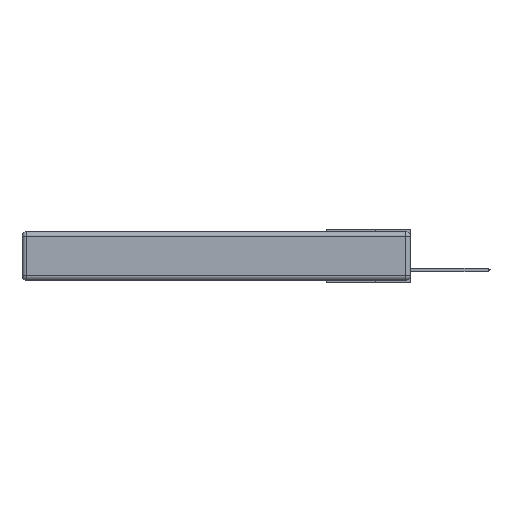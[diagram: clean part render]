
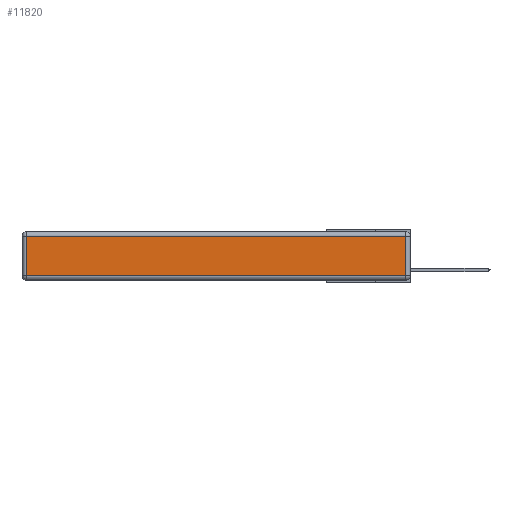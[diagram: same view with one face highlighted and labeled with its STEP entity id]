
A CAD part, left-side view. The second image highlights one B-rep face of the part: STEP entity #11820.
In plain terms, the highlighted planar face has unit normal (-1, 0, 0).
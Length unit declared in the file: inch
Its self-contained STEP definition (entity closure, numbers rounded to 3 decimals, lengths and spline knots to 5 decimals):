
#260 = VECTOR ( 'NONE', #11265, 39.37008 ) ;
#859 = CARTESIAN_POINT ( 'NONE',  ( 0., 0., -0.343 ) ) ;
#1187 = ORIENTED_EDGE ( 'NONE', *, *, #10939, .T. ) ;
#1358 = VECTOR ( 'NONE', #7490, 39.37008 ) ;
#1414 = CARTESIAN_POINT ( 'NONE',  ( 0., 2.72, -0.313 ) ) ;
#1462 = VERTEX_POINT ( 'NONE', #13687 ) ;
#1699 = LINE ( 'NONE', #4049, #10821 ) ;
#2009 = VERTEX_POINT ( 'NONE', #2602 ) ;
#2602 = CARTESIAN_POINT ( 'NONE',  ( 0., 0.03, -0.03 ) ) ;
#2929 = EDGE_CURVE ( 'NONE', #2009, #7549, #1699, .T. ) ;
#3170 = DIRECTION ( 'NONE',  ( -1., 0., 0. ) ) ;
#3746 = DIRECTION ( 'NONE',  ( 0., -1., 0. ) ) ;
#4049 = CARTESIAN_POINT ( 'NONE',  ( 0., 2.75, -0.03 ) ) ;
#4185 = ORIENTED_EDGE ( 'NONE', *, *, #13434, .T. ) ;
#4400 = VERTEX_POINT ( 'NONE', #1414 ) ;
#4493 = AXIS2_PLACEMENT_3D ( 'NONE', #859, #3170, #6265 ) ;
#4507 = VECTOR ( 'NONE', #3746, 39.37008 ) ;
#5221 = DIRECTION ( 'NONE',  ( 0., 1., 0. ) ) ;
#5740 = ORIENTED_EDGE ( 'NONE', *, *, #2929, .T. ) ;
#6265 = DIRECTION ( 'NONE',  ( 0., 0., 1. ) ) ;
#6536 = CARTESIAN_POINT ( 'NONE',  ( 0., 0.03, -0.343 ) ) ;
#6950 = ORIENTED_EDGE ( 'NONE', *, *, #8237, .T. ) ;
#7490 = DIRECTION ( 'NONE',  ( 0., 0., -1. ) ) ;
#7549 = VERTEX_POINT ( 'NONE', #8307 ) ;
#7994 = LINE ( 'NONE', #11583, #1358 ) ;
#8237 = EDGE_CURVE ( 'NONE', #4400, #1462, #10099, .T. ) ;
#8307 = CARTESIAN_POINT ( 'NONE',  ( 0., 2.72, -0.03 ) ) ;
#9371 = LINE ( 'NONE', #6536, #260 ) ;
#9476 = PLANE ( 'NONE',  #4493 ) ;
#9855 = FACE_OUTER_BOUND ( 'NONE', #12672, .T. ) ;
#10099 = LINE ( 'NONE', #11098, #4507 ) ;
#10821 = VECTOR ( 'NONE', #5221, 39.37008 ) ;
#10939 = EDGE_CURVE ( 'NONE', #1462, #2009, #9371, .T. ) ;
#11098 = CARTESIAN_POINT ( 'NONE',  ( 0., 0., -0.313 ) ) ;
#11265 = DIRECTION ( 'NONE',  ( 0., 0., 1. ) ) ;
#11583 = CARTESIAN_POINT ( 'NONE',  ( 0., 2.72, -0.343 ) ) ;
#11820 = ADVANCED_FACE ( 'NONE', ( #9855 ), #9476, .T. ) ;
#12672 = EDGE_LOOP ( 'NONE', ( #6950, #1187, #5740, #4185 ) ) ;
#13434 = EDGE_CURVE ( 'NONE', #7549, #4400, #7994, .T. ) ;
#13687 = CARTESIAN_POINT ( 'NONE',  ( 0., 0.03, -0.313 ) ) ;
